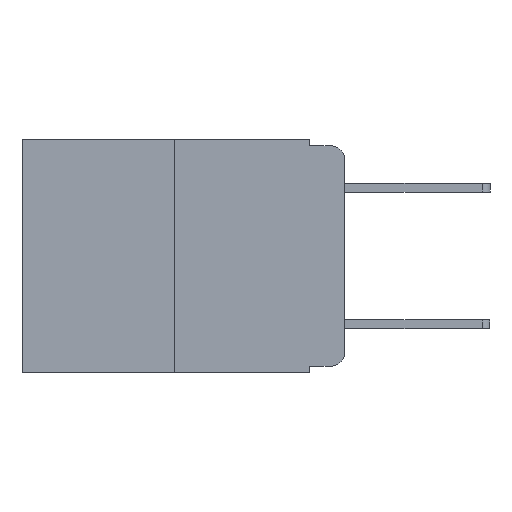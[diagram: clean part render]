
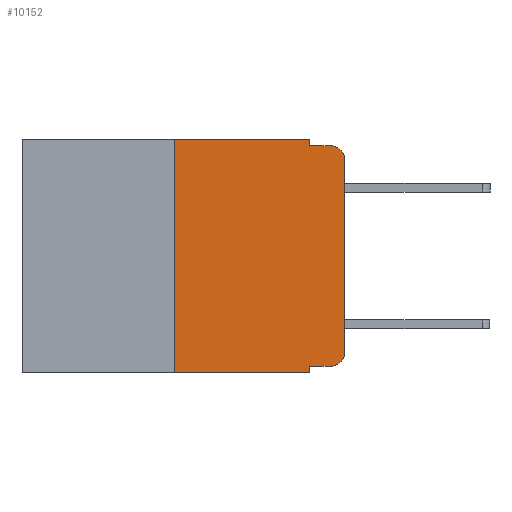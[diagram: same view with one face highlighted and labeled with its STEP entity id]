
A CAD part, left-side view. The second image highlights one B-rep face of the part: STEP entity #10152.
In plain terms, the highlighted planar face has unit normal (-1, 0, 0).
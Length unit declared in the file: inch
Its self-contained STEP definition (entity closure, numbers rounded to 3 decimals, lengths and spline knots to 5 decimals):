
#13 = LINE ( 'NONE', #12041, #17838 ) ;
#274 = CARTESIAN_POINT ( 'NONE',  ( 0., 0.051, -0.01 ) ) ;
#281 = VERTEX_POINT ( 'NONE', #14682 ) ;
#357 = DIRECTION ( 'NONE',  ( 0., 0., -1. ) ) ;
#423 = DIRECTION ( 'NONE',  ( 0., -1., 0. ) ) ;
#491 = VERTEX_POINT ( 'NONE', #16281 ) ;
#611 = DIRECTION ( 'NONE',  ( 0., 0., -1. ) ) ;
#1615 = LINE ( 'NONE', #13215, #8755 ) ;
#1713 = CARTESIAN_POINT ( 'NONE',  ( 0., 0.051, -0.01 ) ) ;
#1966 = VERTEX_POINT ( 'NONE', #5272 ) ;
#1989 = ORIENTED_EDGE ( 'NONE', *, *, #4279, .F. ) ;
#2054 = CARTESIAN_POINT ( 'NONE',  ( 0., 0.051, 0. ) ) ;
#2116 = ORIENTED_EDGE ( 'NONE', *, *, #4275, .F. ) ;
#2145 = ORIENTED_EDGE ( 'NONE', *, *, #3477, .F. ) ;
#3430 = LINE ( 'NONE', #17270, #10633 ) ;
#3477 = EDGE_CURVE ( 'NONE', #9391, #16248, #5202, .T. ) ;
#3563 = CARTESIAN_POINT ( 'NONE',  ( 0., 0.02, -0.03 ) ) ;
#3734 = VERTEX_POINT ( 'NONE', #1713 ) ;
#3880 = DIRECTION ( 'NONE',  ( 0., -1., 0. ) ) ;
#3948 = EDGE_CURVE ( 'NONE', #491, #1966, #13052, .T. ) ;
#4073 = ORIENTED_EDGE ( 'NONE', *, *, #4253, .T. ) ;
#4139 = ORIENTED_EDGE ( 'NONE', *, *, #4305, .F. ) ;
#4180 = CARTESIAN_POINT ( 'NONE',  ( 0., 0.25, 0. ) ) ;
#4190 = FACE_OUTER_BOUND ( 'NONE', #11289, .T. ) ;
#4250 = EDGE_CURVE ( 'NONE', #5981, #281, #1615, .T. ) ;
#4253 = EDGE_CURVE ( 'NONE', #281, #14037, #12223, .T. ) ;
#4275 = EDGE_CURVE ( 'NONE', #3734, #14037, #11820, .T. ) ;
#4279 = EDGE_CURVE ( 'NONE', #16248, #3734, #8319, .T. ) ;
#4284 = EDGE_CURVE ( 'NONE', #491, #9391, #13, .T. ) ;
#4305 = EDGE_CURVE ( 'NONE', #9219, #1966, #7414, .T. ) ;
#4308 = EDGE_CURVE ( 'NONE', #9219, #15236, #3430, .T. ) ;
#4309 = EDGE_CURVE ( 'NONE', #15236, #5981, #14032, .T. ) ;
#4438 = VECTOR ( 'NONE', #10775, 39.37008 ) ;
#5144 = DIRECTION ( 'NONE',  ( 0., 0., -1. ) ) ;
#5202 = LINE ( 'NONE', #14837, #8583 ) ;
#5272 = CARTESIAN_POINT ( 'NONE',  ( 0., 0.051, -0.343 ) ) ;
#5343 = DIRECTION ( 'NONE',  ( -1., 0., 0. ) ) ;
#5961 = ORIENTED_EDGE ( 'NONE', *, *, #4308, .T. ) ;
#5981 = VERTEX_POINT ( 'NONE', #8992 ) ;
#6255 = ORIENTED_EDGE ( 'NONE', *, *, #4309, .T. ) ;
#6662 = ORIENTED_EDGE ( 'NONE', *, *, #3948, .T. ) ;
#6839 = ORIENTED_EDGE ( 'NONE', *, *, #4284, .F. ) ;
#6882 = PLANE ( 'NONE',  #13733 ) ;
#7414 = LINE ( 'NONE', #2054, #17444 ) ;
#7872 = VECTOR ( 'NONE', #14635, 39.37008 ) ;
#7991 = DIRECTION ( 'NONE',  ( 0., 0., 1. ) ) ;
#8124 = DIRECTION ( 'NONE',  ( 0., 0., 1. ) ) ;
#8290 = CARTESIAN_POINT ( 'NONE',  ( 0., 0.051, -0.333 ) ) ;
#8319 = LINE ( 'NONE', #14583, #7872 ) ;
#8583 = VECTOR ( 'NONE', #3880, 39.37008 ) ;
#8755 = VECTOR ( 'NONE', #7991, 39.37008 ) ;
#8992 = CARTESIAN_POINT ( 'NONE',  ( 0., 0., -0.313 ) ) ;
#9219 = VERTEX_POINT ( 'NONE', #8290 ) ;
#9391 = VERTEX_POINT ( 'NONE', #4180 ) ;
#9707 = DIRECTION ( 'NONE',  ( 1., 0., 0. ) ) ;
#9870 = CARTESIAN_POINT ( 'NONE',  ( 0., 0.473, -0.343 ) ) ;
#10152 = ADVANCED_FACE ( 'NONE', ( #4190 ), #6882, .F. ) ;
#10167 = CARTESIAN_POINT ( 'NONE',  ( 0., 0.02, -0.01 ) ) ;
#10633 = VECTOR ( 'NONE', #423, 39.37008 ) ;
#10775 = DIRECTION ( 'NONE',  ( 0., -1., 0. ) ) ;
#10925 = CARTESIAN_POINT ( 'NONE',  ( 0., 0.02, -0.333 ) ) ;
#11289 = EDGE_LOOP ( 'NONE', ( #14767, #4073, #2116, #1989, #2145, #6839, #6662, #4139, #5961, #6255 ) ) ;
#11820 = LINE ( 'NONE', #274, #4438 ) ;
#12041 = CARTESIAN_POINT ( 'NONE',  ( 0., 0.25, 0. ) ) ;
#12223 = CIRCLE ( 'NONE', #13144, 0.02 ) ;
#12243 = VECTOR ( 'NONE', #16340, 39.37008 ) ;
#13052 = LINE ( 'NONE', #9870, #12243 ) ;
#13144 = AXIS2_PLACEMENT_3D ( 'NONE', #3563, #13278, #5144 ) ;
#13215 = CARTESIAN_POINT ( 'NONE',  ( 0., 0., 0. ) ) ;
#13278 = DIRECTION ( 'NONE',  ( -1., 0., 0. ) ) ;
#13442 = CARTESIAN_POINT ( 'NONE',  ( 0., 0.02, -0.313 ) ) ;
#13733 = AXIS2_PLACEMENT_3D ( 'NONE', #17398, #9707, #611 ) ;
#13801 = CARTESIAN_POINT ( 'NONE',  ( 0., 0.051, 0. ) ) ;
#14032 = CIRCLE ( 'NONE', #17456, 0.02 ) ;
#14037 = VERTEX_POINT ( 'NONE', #10167 ) ;
#14583 = CARTESIAN_POINT ( 'NONE',  ( 0., 0.051, 0. ) ) ;
#14635 = DIRECTION ( 'NONE',  ( 0., 0., -1. ) ) ;
#14682 = CARTESIAN_POINT ( 'NONE',  ( 0., 0., -0.03 ) ) ;
#14746 = DIRECTION ( 'NONE',  ( 0., 0., -1. ) ) ;
#14767 = ORIENTED_EDGE ( 'NONE', *, *, #4250, .T. ) ;
#14837 = CARTESIAN_POINT ( 'NONE',  ( 0., 0.473, 0. ) ) ;
#15236 = VERTEX_POINT ( 'NONE', #10925 ) ;
#16248 = VERTEX_POINT ( 'NONE', #13801 ) ;
#16281 = CARTESIAN_POINT ( 'NONE',  ( 0., 0.25, -0.343 ) ) ;
#16340 = DIRECTION ( 'NONE',  ( 0., -1., 0. ) ) ;
#17270 = CARTESIAN_POINT ( 'NONE',  ( 0., 0.051, -0.333 ) ) ;
#17398 = CARTESIAN_POINT ( 'NONE',  ( 0., 0.473, 0. ) ) ;
#17444 = VECTOR ( 'NONE', #357, 39.37008 ) ;
#17456 = AXIS2_PLACEMENT_3D ( 'NONE', #13442, #5343, #14746 ) ;
#17838 = VECTOR ( 'NONE', #8124, 39.37008 ) ;
